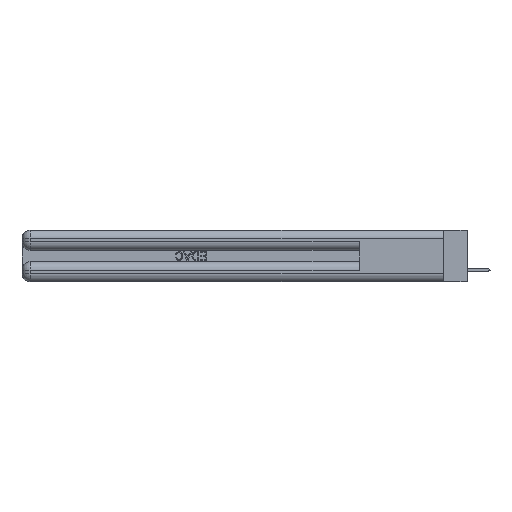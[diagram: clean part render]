
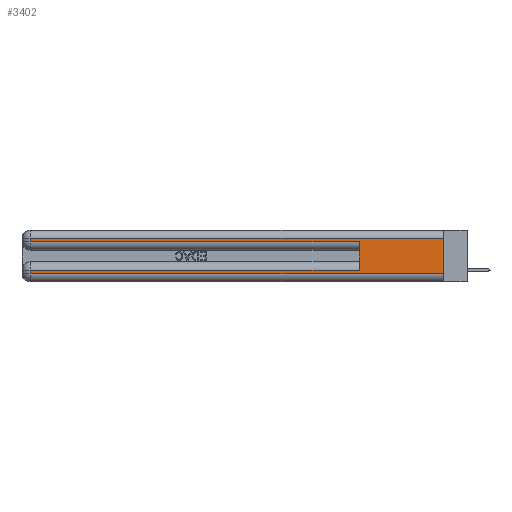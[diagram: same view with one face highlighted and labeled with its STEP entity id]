
A CAD part, left-side view. The second image highlights one B-rep face of the part: STEP entity #3402.
In plain terms, the highlighted planar face has unit normal (-1, 0, 0).
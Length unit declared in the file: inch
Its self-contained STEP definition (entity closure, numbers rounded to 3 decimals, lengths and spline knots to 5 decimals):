
#258 = ORIENTED_EDGE ( 'NONE', *, *, #8162, .T. ) ;
#472 = CARTESIAN_POINT ( 'NONE',  ( 0., 0., 0.31 ) ) ;
#669 = VECTOR ( 'NONE', #2533, 39.37008 ) ;
#754 = DIRECTION ( 'NONE',  ( 0., 1., 0. ) ) ;
#1195 = LINE ( 'NONE', #19775, #23377 ) ;
#1522 = CARTESIAN_POINT ( 'NONE',  ( 0., 0., 0.06 ) ) ;
#1791 = DIRECTION ( 'NONE',  ( 1., 0., 0. ) ) ;
#1923 = AXIS2_PLACEMENT_3D ( 'NONE', #23966, #1791, #14993 ) ;
#2119 = VECTOR ( 'NONE', #13509, 39.37008 ) ;
#2225 = CARTESIAN_POINT ( 'NONE',  ( 0., 0., 0.085 ) ) ;
#2525 = DIRECTION ( 'NONE',  ( 0., -1., 0. ) ) ;
#2533 = DIRECTION ( 'NONE',  ( 0., 0., -1. ) ) ;
#2968 = VERTEX_POINT ( 'NONE', #12325 ) ;
#3402 = ADVANCED_FACE ( 'NONE', ( #39116 ), #36756, .F. ) ;
#3980 = VECTOR ( 'NONE', #754, 39.37008 ) ;
#4534 = ORIENTED_EDGE ( 'NONE', *, *, #7117, .T. ) ;
#4568 = DIRECTION ( 'NONE',  ( 0., 0., -1. ) ) ;
#5804 = CARTESIAN_POINT ( 'NONE',  ( 0., 0.6, 0.145 ) ) ;
#6929 = EDGE_CURVE ( 'NONE', #34392, #33288, #13666, .T. ) ;
#7117 = EDGE_CURVE ( 'NONE', #32923, #33288, #1195, .T. ) ;
#7309 = LINE ( 'NONE', #11862, #31488 ) ;
#8162 = EDGE_CURVE ( 'NONE', #22569, #32923, #7309, .T. ) ;
#8597 = CARTESIAN_POINT ( 'NONE',  ( 0., 2.94, 0.085 ) ) ;
#9031 = VERTEX_POINT ( 'NONE', #21838 ) ;
#10445 = VECTOR ( 'NONE', #32354, 39.37008 ) ;
#11862 = CARTESIAN_POINT ( 'NONE',  ( 0., 2.94, 0.37 ) ) ;
#12325 = CARTESIAN_POINT ( 'NONE',  ( 0., 2.94, 0.285 ) ) ;
#13013 = ORIENTED_EDGE ( 'NONE', *, *, #6929, .F. ) ;
#13509 = DIRECTION ( 'NONE',  ( 0., -1., 0. ) ) ;
#13666 = LINE ( 'NONE', #14982, #669 ) ;
#14305 = VECTOR ( 'NONE', #16950, 39.37008 ) ;
#14368 = LINE ( 'NONE', #472, #3980 ) ;
#14982 = CARTESIAN_POINT ( 'NONE',  ( 0., 0., 0.37 ) ) ;
#14993 = DIRECTION ( 'NONE',  ( 0., 0., -1. ) ) ;
#15587 = CARTESIAN_POINT ( 'NONE',  ( 0., 0.6, 0.285 ) ) ;
#16950 = DIRECTION ( 'NONE',  ( 0., 0., -1. ) ) ;
#18209 = EDGE_LOOP ( 'NONE', ( #13013, #39666, #28556, #27447, #22865, #29452, #258, #4534 ) ) ;
#18990 = LINE ( 'NONE', #36561, #14305 ) ;
#19480 = LINE ( 'NONE', #2225, #41475 ) ;
#19775 = CARTESIAN_POINT ( 'NONE',  ( 0., 0., 0.06 ) ) ;
#21838 = CARTESIAN_POINT ( 'NONE',  ( 0., 2.94, 0.31 ) ) ;
#22246 = EDGE_CURVE ( 'NONE', #2968, #24940, #29411, .T. ) ;
#22569 = VERTEX_POINT ( 'NONE', #8597 ) ;
#22865 = ORIENTED_EDGE ( 'NONE', *, *, #34835, .F. ) ;
#23377 = VECTOR ( 'NONE', #2525, 39.37008 ) ;
#23590 = CARTESIAN_POINT ( 'NONE',  ( 0., 0., 0.31 ) ) ;
#23966 = CARTESIAN_POINT ( 'NONE',  ( 0., 0., 0.37 ) ) ;
#24859 = LINE ( 'NONE', #5804, #10445 ) ;
#24940 = VERTEX_POINT ( 'NONE', #15587 ) ;
#25242 = EDGE_CURVE ( 'NONE', #9031, #2968, #18990, .T. ) ;
#25550 = EDGE_CURVE ( 'NONE', #42352, #22569, #19480, .T. ) ;
#27447 = ORIENTED_EDGE ( 'NONE', *, *, #22246, .T. ) ;
#28556 = ORIENTED_EDGE ( 'NONE', *, *, #25242, .T. ) ;
#29034 = EDGE_CURVE ( 'NONE', #34392, #9031, #14368, .T. ) ;
#29411 = LINE ( 'NONE', #36803, #2119 ) ;
#29452 = ORIENTED_EDGE ( 'NONE', *, *, #25550, .T. ) ;
#31488 = VECTOR ( 'NONE', #4568, 39.37008 ) ;
#32354 = DIRECTION ( 'NONE',  ( 0., 0., 1. ) ) ;
#32923 = VERTEX_POINT ( 'NONE', #36894 ) ;
#33288 = VERTEX_POINT ( 'NONE', #1522 ) ;
#34392 = VERTEX_POINT ( 'NONE', #23590 ) ;
#34835 = EDGE_CURVE ( 'NONE', #42352, #24940, #24859, .T. ) ;
#35816 = DIRECTION ( 'NONE',  ( 0., 1., 0. ) ) ;
#36561 = CARTESIAN_POINT ( 'NONE',  ( 0., 2.94, 0.37 ) ) ;
#36756 = PLANE ( 'NONE',  #1923 ) ;
#36803 = CARTESIAN_POINT ( 'NONE',  ( 0., 0., 0.285 ) ) ;
#36894 = CARTESIAN_POINT ( 'NONE',  ( 0., 2.94, 0.06 ) ) ;
#39116 = FACE_OUTER_BOUND ( 'NONE', #18209, .T. ) ;
#39666 = ORIENTED_EDGE ( 'NONE', *, *, #29034, .T. ) ;
#41475 = VECTOR ( 'NONE', #35816, 39.37008 ) ;
#42352 = VERTEX_POINT ( 'NONE', #42524 ) ;
#42524 = CARTESIAN_POINT ( 'NONE',  ( 0., 0.6, 0.085 ) ) ;
